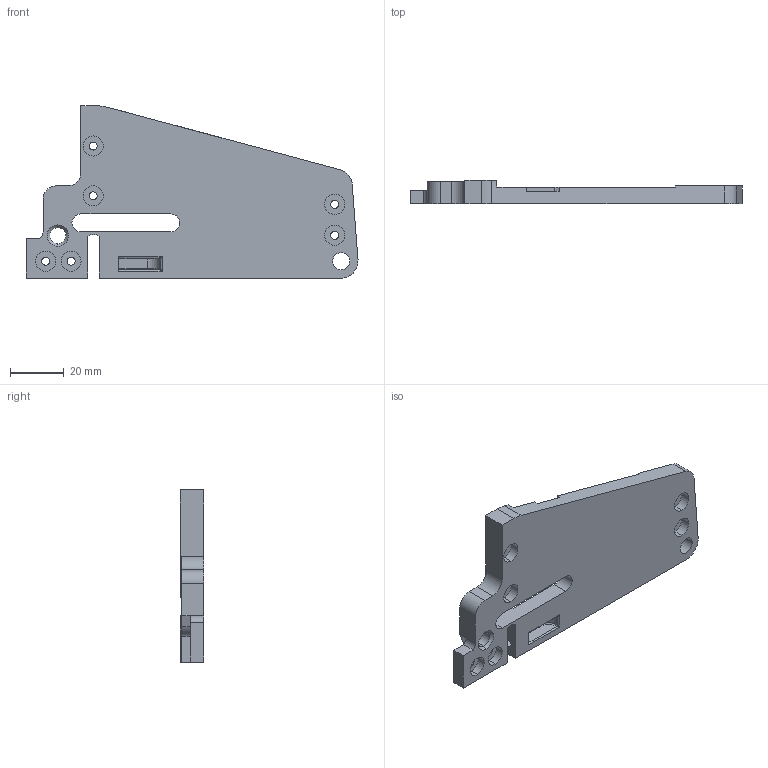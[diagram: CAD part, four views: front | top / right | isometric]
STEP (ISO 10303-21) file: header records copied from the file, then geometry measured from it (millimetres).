
FILE_DESCRIPTION (( 'STEP AP214' ), '1' );
FILE_NAME ('Thunderbolt_Mag_Well_Left_Blank.STEP', '2021-09-12T03:34:04', ( '' ), ( '' ), 'SwSTEP 2.0', 'SolidWorks 2020', '' );
FILE_SCHEMA (( 'AUTOMOTIVE_DESIGN' ));
Length unit declared in the file: millimetre
Products named in the file (1): Thunderbolt_Mag_Well_Left_Blank
Bounding box: 124.06 x 8.75 x 64.36 mm (x, y, z)
Volume: 34896.9 mm3; surface area: 15858.6 mm2
Topology: 1 solids, 1 shells, 131 faces, 341 edges, 213 vertices
Faces by surface type: cylinder 57, plane 56, bspline 11, sphere 3, cone 2, torus 2
Entity records: 4191 total; most frequent: CARTESIAN_POINT 987, ORIENTED_EDGE 672, DIRECTION 649, EDGE_CURVE 336, AXIS2_PLACEMENT_3D 227, VERTEX_POINT 213, VECTOR 195, LINE 195
